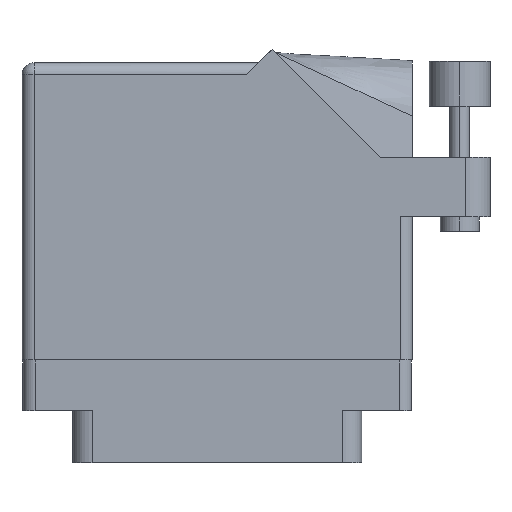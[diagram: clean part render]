
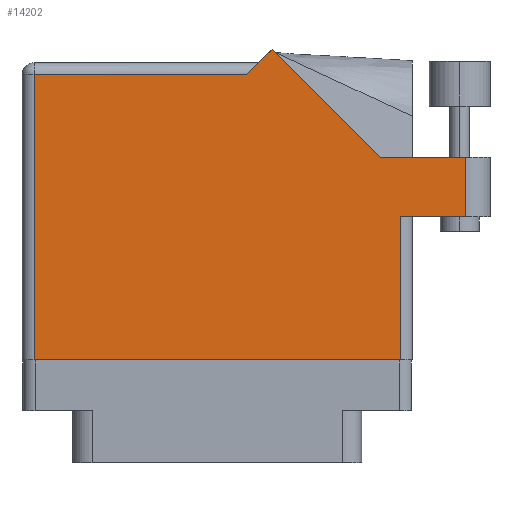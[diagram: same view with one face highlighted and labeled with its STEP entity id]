
A CAD part, front view. The second image highlights one B-rep face of the part: STEP entity #14202.
In plain terms, the highlighted face is planar.
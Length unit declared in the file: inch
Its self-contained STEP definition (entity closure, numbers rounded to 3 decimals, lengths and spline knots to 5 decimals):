
#497 = CARTESIAN_POINT ( 'NONE',  ( 1.217, 1.53, 0. ) ) ;
#1412 = EDGE_CURVE ( 'NONE', #25951, #13105, #35083, .T. ) ;
#1461 = LINE ( 'NONE', #33582, #2728 ) ;
#1830 = DIRECTION ( 'NONE',  ( 1., 0., 0. ) ) ;
#2384 = VECTOR ( 'NONE', #12851, 39.37008 ) ;
#2728 = VECTOR ( 'NONE', #3910, 39.37008 ) ;
#2747 = CARTESIAN_POINT ( 'NONE',  ( 2.285, 1.044, 0. ) ) ;
#3060 = LINE ( 'NONE', #6853, #12408 ) ;
#3383 = EDGE_CURVE ( 'NONE', #6124, #19609, #3060, .T. ) ;
#3910 = DIRECTION ( 'NONE',  ( -0.707, 0.707, 0. ) ) ;
#4290 = VERTEX_POINT ( 'NONE', #6554 ) ;
#4930 = DIRECTION ( 'NONE',  ( 0., 0., -1. ) ) ;
#6124 = VERTEX_POINT ( 'NONE', #29592 ) ;
#6554 = CARTESIAN_POINT ( 'NONE',  ( 0.062, 1.468, 0. ) ) ;
#6842 = DIRECTION ( 'NONE',  ( 0., 1., 0. ) ) ;
#6853 = CARTESIAN_POINT ( 'NONE',  ( 2.01, 0.737, 0. ) ) ;
#6884 = ORIENTED_EDGE ( 'NONE', *, *, #24055, .T. ) ;
#7060 = EDGE_CURVE ( 'NONE', #13105, #4290, #21054, .T. ) ;
#7074 = CARTESIAN_POINT ( 'NONE',  ( 1.28771, 1.60071, 0. ) ) ;
#7407 = CARTESIAN_POINT ( 'NONE',  ( 0.062, 0., 0. ) ) ;
#8519 = CARTESIAN_POINT ( 'NONE',  ( 2.41, 1.044, 0. ) ) ;
#9537 = VECTOR ( 'NONE', #6842, 39.37008 ) ;
#9612 = CARTESIAN_POINT ( 'NONE',  ( 1.155, 1.468, 0. ) ) ;
#10374 = DIRECTION ( 'NONE',  ( -1., 0., 0. ) ) ;
#10909 = VECTOR ( 'NONE', #30041, 39.37008 ) ;
#12408 = VECTOR ( 'NONE', #1830, 39.37008 ) ;
#12851 = DIRECTION ( 'NONE',  ( 1., 0., 0. ) ) ;
#13105 = VERTEX_POINT ( 'NONE', #9612 ) ;
#13146 = EDGE_CURVE ( 'NONE', #32453, #27753, #28917, .T. ) ;
#13788 = LINE ( 'NONE', #17520, #22205 ) ;
#14202 = ADVANCED_FACE ( 'NONE', ( #28853 ), #31860, .F. ) ;
#14351 = DIRECTION ( 'NONE',  ( -0.707, -0.707, 0. ) ) ;
#15537 = EDGE_CURVE ( 'NONE', #4290, #16959, #13788, .T. ) ;
#15683 = CARTESIAN_POINT ( 'NONE',  ( 0., 1.53, 0. ) ) ;
#16056 = VECTOR ( 'NONE', #14351, 39.37008 ) ;
#16234 = EDGE_CURVE ( 'NONE', #19609, #32453, #17106, .T. ) ;
#16344 = ORIENTED_EDGE ( 'NONE', *, *, #23096, .T. ) ;
#16486 = EDGE_LOOP ( 'NONE', ( #31620, #24793, #30315, #6884, #32612, #27359, #34521, #16344, #32761 ) ) ;
#16959 = VERTEX_POINT ( 'NONE', #7407 ) ;
#17106 = LINE ( 'NONE', #33537, #9537 ) ;
#17520 = CARTESIAN_POINT ( 'NONE',  ( 0.062, 0., 0. ) ) ;
#18708 = CARTESIAN_POINT ( 'NONE',  ( 1.948, 0., 0. ) ) ;
#19609 = VERTEX_POINT ( 'NONE', #31781 ) ;
#21054 = LINE ( 'NONE', #27395, #10909 ) ;
#21488 = DIRECTION ( 'NONE',  ( -1., 0., 0. ) ) ;
#22205 = VECTOR ( 'NONE', #27775, 39.37008 ) ;
#23096 = EDGE_CURVE ( 'NONE', #16959, #32247, #27743, .T. ) ;
#24055 = EDGE_CURVE ( 'NONE', #27753, #25951, #1461, .T. ) ;
#24793 = ORIENTED_EDGE ( 'NONE', *, *, #16234, .T. ) ;
#25613 = LINE ( 'NONE', #29301, #33251 ) ;
#25951 = VERTEX_POINT ( 'NONE', #7074 ) ;
#26412 = CARTESIAN_POINT ( 'NONE',  ( 0., 0., 0. ) ) ;
#27359 = ORIENTED_EDGE ( 'NONE', *, *, #7060, .T. ) ;
#27395 = CARTESIAN_POINT ( 'NONE',  ( 0., 1.468, 0. ) ) ;
#27743 = LINE ( 'NONE', #26412, #2384 ) ;
#27753 = VERTEX_POINT ( 'NONE', #31400 ) ;
#27775 = DIRECTION ( 'NONE',  ( 0., -1., 0. ) ) ;
#28853 = FACE_OUTER_BOUND ( 'NONE', #16486, .T. ) ;
#28917 = LINE ( 'NONE', #8519, #34847 ) ;
#29301 = CARTESIAN_POINT ( 'NONE',  ( 1.948, 0.737, 0. ) ) ;
#29592 = CARTESIAN_POINT ( 'NONE',  ( 1.948, 0.737, 0. ) ) ;
#30041 = DIRECTION ( 'NONE',  ( -1., 0., 0. ) ) ;
#30315 = ORIENTED_EDGE ( 'NONE', *, *, #13146, .T. ) ;
#31400 = CARTESIAN_POINT ( 'NONE',  ( 1.84442, 1.044, 0. ) ) ;
#31403 = AXIS2_PLACEMENT_3D ( 'NONE', #15683, #4930, #10374 ) ;
#31620 = ORIENTED_EDGE ( 'NONE', *, *, #3383, .T. ) ;
#31781 = CARTESIAN_POINT ( 'NONE',  ( 2.285, 0.737, 0. ) ) ;
#31860 = PLANE ( 'NONE',  #31403 ) ;
#32247 = VERTEX_POINT ( 'NONE', #18708 ) ;
#32453 = VERTEX_POINT ( 'NONE', #2747 ) ;
#32612 = ORIENTED_EDGE ( 'NONE', *, *, #1412, .T. ) ;
#32761 = ORIENTED_EDGE ( 'NONE', *, *, #33341, .T. ) ;
#33251 = VECTOR ( 'NONE', #34254, 39.37008 ) ;
#33341 = EDGE_CURVE ( 'NONE', #32247, #6124, #25613, .T. ) ;
#33537 = CARTESIAN_POINT ( 'NONE',  ( 2.285, 1.044, 0. ) ) ;
#33582 = CARTESIAN_POINT ( 'NONE',  ( 1.84442, 1.044, 0. ) ) ;
#34254 = DIRECTION ( 'NONE',  ( 0., 1., 0. ) ) ;
#34521 = ORIENTED_EDGE ( 'NONE', *, *, #15537, .T. ) ;
#34847 = VECTOR ( 'NONE', #21488, 39.37008 ) ;
#35083 = LINE ( 'NONE', #497, #16056 ) ;
